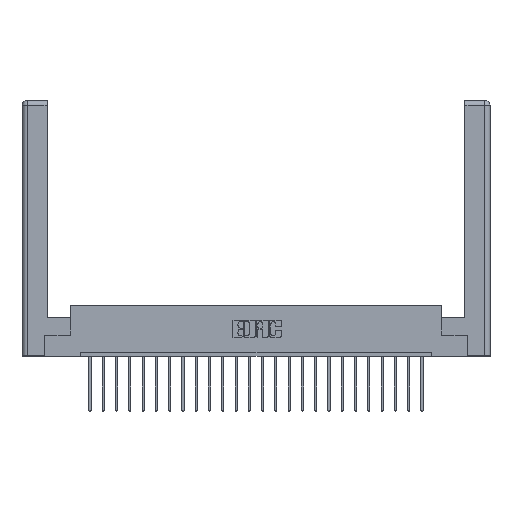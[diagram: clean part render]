
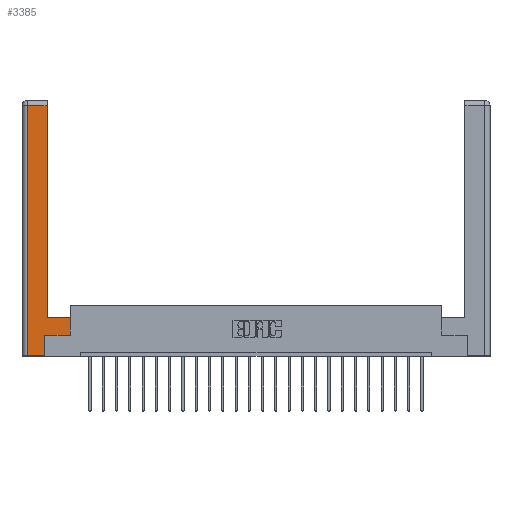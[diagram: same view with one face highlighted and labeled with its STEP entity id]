
A CAD part, top view. The second image highlights one B-rep face of the part: STEP entity #3385.
In plain terms, the highlighted planar face has unit normal (0, 0, 1).
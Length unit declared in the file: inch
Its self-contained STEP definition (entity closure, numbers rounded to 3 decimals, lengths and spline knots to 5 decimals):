
#78 = VECTOR ( 'NONE', #7773, 39.37008 ) ;
#367 = PLANE ( 'NONE',  #16006 ) ;
#2014 = VECTOR ( 'NONE', #14901, 39.37008 ) ;
#2162 = DIRECTION ( 'NONE',  ( -1., 0., 0. ) ) ;
#3183 = CARTESIAN_POINT ( 'NONE',  ( 0.565, 0.245, 0. ) ) ;
#3239 = CARTESIAN_POINT ( 'NONE',  ( 0.0615, 2.94, 0. ) ) ;
#3385 = ADVANCED_FACE ( 'NONE', ( #14066 ), #367, .F. ) ;
#3536 = VERTEX_POINT ( 'NONE', #17786 ) ;
#3624 = CARTESIAN_POINT ( 'NONE',  ( 0.295, 0.45, 0. ) ) ;
#3790 = ORIENTED_EDGE ( 'NONE', *, *, #9841, .T. ) ;
#3860 = CARTESIAN_POINT ( 'NONE',  ( 0.0615, 0., 0. ) ) ;
#3866 = VECTOR ( 'NONE', #6679, 39.37008 ) ;
#4680 = EDGE_CURVE ( 'NONE', #23999, #3536, #16778, .T. ) ;
#4768 = LINE ( 'NONE', #3860, #78 ) ;
#5317 = CARTESIAN_POINT ( 'NONE',  ( 0.265, 0., 0. ) ) ;
#5435 = VERTEX_POINT ( 'NONE', #3239 ) ;
#5723 = VECTOR ( 'NONE', #10918, 39.37008 ) ;
#5822 = CARTESIAN_POINT ( 'NONE',  ( 0.265, 0.245, 0. ) ) ;
#6249 = ORIENTED_EDGE ( 'NONE', *, *, #21349, .T. ) ;
#6679 = DIRECTION ( 'NONE',  ( 0., 1., 0. ) ) ;
#6985 = DIRECTION ( 'NONE',  ( 0., 1., 0. ) ) ;
#7773 = DIRECTION ( 'NONE',  ( 0., -1., 0. ) ) ;
#7826 = VECTOR ( 'NONE', #13371, 39.37008 ) ;
#8016 = EDGE_CURVE ( 'NONE', #15985, #5435, #10628, .T. ) ;
#9841 = EDGE_CURVE ( 'NONE', #5435, #23999, #4768, .T. ) ;
#10628 = LINE ( 'NONE', #18606, #11235 ) ;
#10918 = DIRECTION ( 'NONE',  ( 1., 0., 0. ) ) ;
#11235 = VECTOR ( 'NONE', #22304, 39.37008 ) ;
#11242 = EDGE_LOOP ( 'NONE', ( #13049, #16804, #3790, #13095, #6249, #22269, #12484, #22085 ) ) ;
#11610 = DIRECTION ( 'NONE',  ( 0., 0., -1. ) ) ;
#11666 = LINE ( 'NONE', #19869, #15745 ) ;
#12484 = ORIENTED_EDGE ( 'NONE', *, *, #23285, .T. ) ;
#12618 = CARTESIAN_POINT ( 'NONE',  ( 0.565, 0.245, 0. ) ) ;
#12881 = VERTEX_POINT ( 'NONE', #13785 ) ;
#13049 = ORIENTED_EDGE ( 'NONE', *, *, #16331, .T. ) ;
#13095 = ORIENTED_EDGE ( 'NONE', *, *, #4680, .T. ) ;
#13371 = DIRECTION ( 'NONE',  ( 0., 1., 0. ) ) ;
#13785 = CARTESIAN_POINT ( 'NONE',  ( 0.565, 0.45, 0. ) ) ;
#14066 = FACE_OUTER_BOUND ( 'NONE', #11242, .T. ) ;
#14901 = DIRECTION ( 'NONE',  ( -1., 0., 0. ) ) ;
#14903 = VERTEX_POINT ( 'NONE', #12618 ) ;
#15368 = CARTESIAN_POINT ( 'NONE',  ( 0.295, 2.94, 0. ) ) ;
#15722 = CARTESIAN_POINT ( 'NONE',  ( 0.0615, 0., 0. ) ) ;
#15745 = VECTOR ( 'NONE', #6985, 39.37008 ) ;
#15919 = VECTOR ( 'NONE', #24007, 39.37008 ) ;
#15985 = VERTEX_POINT ( 'NONE', #15368 ) ;
#15996 = LINE ( 'NONE', #5822, #7826 ) ;
#16006 = AXIS2_PLACEMENT_3D ( 'NONE', #20660, #11610, #2162 ) ;
#16030 = CARTESIAN_POINT ( 'NONE',  ( 0.565, 0.45, 0. ) ) ;
#16331 = EDGE_CURVE ( 'NONE', #16429, #15985, #11666, .T. ) ;
#16429 = VERTEX_POINT ( 'NONE', #3624 ) ;
#16778 = LINE ( 'NONE', #5317, #5723 ) ;
#16804 = ORIENTED_EDGE ( 'NONE', *, *, #8016, .T. ) ;
#17786 = CARTESIAN_POINT ( 'NONE',  ( 0.265, 0., 0. ) ) ;
#18094 = CARTESIAN_POINT ( 'NONE',  ( 0.265, 0.245, 0. ) ) ;
#18606 = CARTESIAN_POINT ( 'NONE',  ( 0.0615, 2.94, 0. ) ) ;
#19526 = VERTEX_POINT ( 'NONE', #18094 ) ;
#19869 = CARTESIAN_POINT ( 'NONE',  ( 0.295, 3., 0. ) ) ;
#20303 = LINE ( 'NONE', #24068, #2014 ) ;
#20660 = CARTESIAN_POINT ( 'NONE',  ( 0., 0., 0. ) ) ;
#21342 = EDGE_CURVE ( 'NONE', #12881, #16429, #20303, .T. ) ;
#21349 = EDGE_CURVE ( 'NONE', #3536, #19526, #15996, .T. ) ;
#21607 = LINE ( 'NONE', #16030, #3866 ) ;
#22085 = ORIENTED_EDGE ( 'NONE', *, *, #21342, .T. ) ;
#22269 = ORIENTED_EDGE ( 'NONE', *, *, #22596, .T. ) ;
#22304 = DIRECTION ( 'NONE',  ( -1., 0., 0. ) ) ;
#22596 = EDGE_CURVE ( 'NONE', #19526, #14903, #23141, .T. ) ;
#23141 = LINE ( 'NONE', #3183, #15919 ) ;
#23285 = EDGE_CURVE ( 'NONE', #14903, #12881, #21607, .T. ) ;
#23999 = VERTEX_POINT ( 'NONE', #15722 ) ;
#24007 = DIRECTION ( 'NONE',  ( 1., 0., 0. ) ) ;
#24068 = CARTESIAN_POINT ( 'NONE',  ( 0.295, 0.45, 0. ) ) ;
